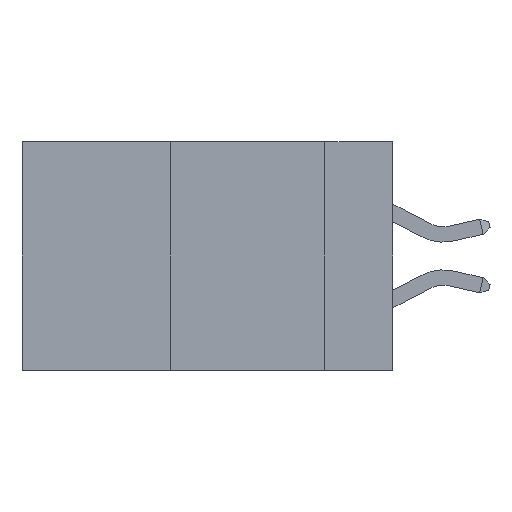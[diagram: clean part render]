
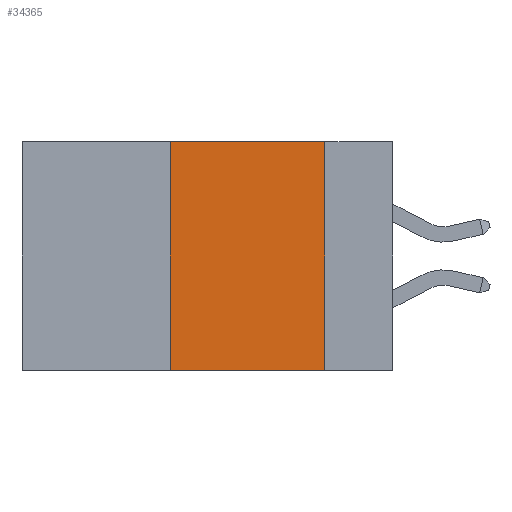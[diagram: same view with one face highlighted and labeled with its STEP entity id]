
A CAD part, left-side view. The second image highlights one B-rep face of the part: STEP entity #34365.
In plain terms, the highlighted planar face has unit normal (-1, 0, 0).
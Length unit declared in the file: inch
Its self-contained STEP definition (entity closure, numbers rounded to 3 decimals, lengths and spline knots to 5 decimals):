
#2183 = EDGE_CURVE ( 'NONE', #26983, #3854, #14660, .T. ) ;
#2833 = DIRECTION ( 'NONE',  ( 1., 0., 0. ) ) ;
#3175 = VERTEX_POINT ( 'NONE', #5974 ) ;
#3854 = VERTEX_POINT ( 'NONE', #31721 ) ;
#4026 = FACE_OUTER_BOUND ( 'NONE', #5266, .T. ) ;
#5266 = EDGE_LOOP ( 'NONE', ( #16948, #26730, #14079, #34455 ) ) ;
#5974 = CARTESIAN_POINT ( 'NONE',  ( 0., 0.36, 0. ) ) ;
#6379 = VERTEX_POINT ( 'NONE', #15437 ) ;
#6641 = EDGE_CURVE ( 'NONE', #6379, #3175, #8023, .T. ) ;
#6758 = DIRECTION ( 'NONE',  ( 0., -1., 0. ) ) ;
#6808 = DIRECTION ( 'NONE',  ( 0., 0., -1. ) ) ;
#8023 = LINE ( 'NONE', #34438, #16884 ) ;
#12054 = EDGE_CURVE ( 'NONE', #6379, #3854, #27971, .T. ) ;
#12331 = CARTESIAN_POINT ( 'NONE',  ( 0., 0.6, -0.37 ) ) ;
#12431 = VECTOR ( 'NONE', #6808, 39.37008 ) ;
#13612 = VECTOR ( 'NONE', #6758, 39.37008 ) ;
#13935 = CARTESIAN_POINT ( 'NONE',  ( 0., 0.6, 0. ) ) ;
#14079 = ORIENTED_EDGE ( 'NONE', *, *, #6641, .F. ) ;
#14660 = LINE ( 'NONE', #14999, #12431 ) ;
#14999 = CARTESIAN_POINT ( 'NONE',  ( 0., 0.11, 0. ) ) ;
#15285 = AXIS2_PLACEMENT_3D ( 'NONE', #13935, #2833, #27874 ) ;
#15437 = CARTESIAN_POINT ( 'NONE',  ( 0., 0.36, -0.37 ) ) ;
#16884 = VECTOR ( 'NONE', #23483, 39.37008 ) ;
#16948 = ORIENTED_EDGE ( 'NONE', *, *, #2183, .F. ) ;
#18618 = VECTOR ( 'NONE', #34398, 39.37008 ) ;
#23483 = DIRECTION ( 'NONE',  ( 0., 0., 1. ) ) ;
#26239 = EDGE_CURVE ( 'NONE', #3175, #26983, #33125, .T. ) ;
#26730 = ORIENTED_EDGE ( 'NONE', *, *, #26239, .F. ) ;
#26983 = VERTEX_POINT ( 'NONE', #31448 ) ;
#27874 = DIRECTION ( 'NONE',  ( 0., 0., -1. ) ) ;
#27971 = LINE ( 'NONE', #12331, #13612 ) ;
#29086 = CARTESIAN_POINT ( 'NONE',  ( 0., 0.6, 0. ) ) ;
#31448 = CARTESIAN_POINT ( 'NONE',  ( 0., 0.11, 0. ) ) ;
#31721 = CARTESIAN_POINT ( 'NONE',  ( 0., 0.11, -0.37 ) ) ;
#33125 = LINE ( 'NONE', #29086, #18618 ) ;
#33801 = PLANE ( 'NONE',  #15285 ) ;
#34365 = ADVANCED_FACE ( 'NONE', ( #4026 ), #33801, .F. ) ;
#34398 = DIRECTION ( 'NONE',  ( 0., -1., 0. ) ) ;
#34438 = CARTESIAN_POINT ( 'NONE',  ( 0., 0.36, 0. ) ) ;
#34455 = ORIENTED_EDGE ( 'NONE', *, *, #12054, .T. ) ;
